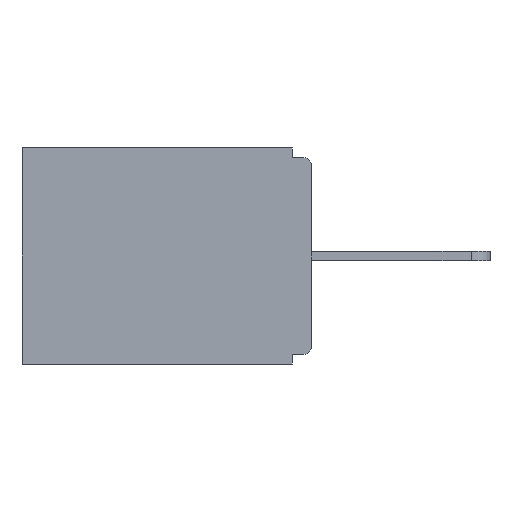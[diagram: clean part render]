
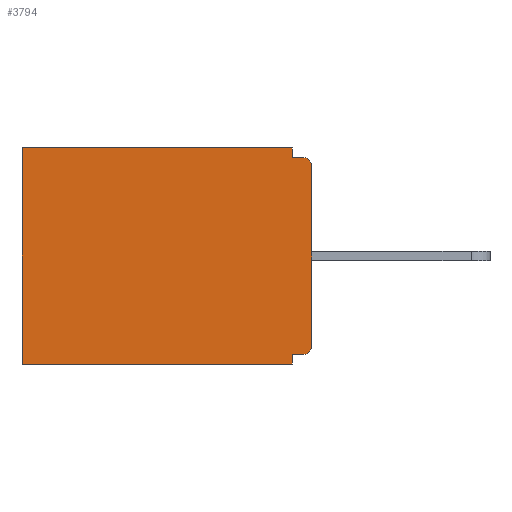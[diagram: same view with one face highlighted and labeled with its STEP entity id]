
A CAD part, left-side view. The second image highlights one B-rep face of the part: STEP entity #3794.
In plain terms, the highlighted planar face has unit normal (-1, 0, 0).
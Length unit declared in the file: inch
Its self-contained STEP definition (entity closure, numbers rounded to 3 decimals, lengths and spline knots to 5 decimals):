
#25 = EDGE_CURVE ( 'NONE', #3244, #3449, #8507, .T. ) ;
#71 = EDGE_CURVE ( 'NONE', #2868, #3944, #8250, .T. ) ;
#76 = EDGE_CURVE ( 'NONE', #2748, #3449, #305, .T. ) ;
#212 = VECTOR ( 'NONE', #11504, 39.37008 ) ;
#305 = CIRCLE ( 'NONE', #8914, 0.015 ) ;
#352 = EDGE_CURVE ( 'NONE', #10212, #10152, #7725, .T. ) ;
#494 = CARTESIAN_POINT ( 'NONE',  ( 0.298, 0., -0.03 ) ) ;
#547 = ORIENTED_EDGE ( 'NONE', *, *, #9572, .F. ) ;
#692 = EDGE_CURVE ( 'NONE', #7930, #3244, #10405, .T. ) ;
#705 = CARTESIAN_POINT ( 'NONE',  ( 0.298, 0.015, -0.015 ) ) ;
#718 = EDGE_CURVE ( 'NONE', #8031, #10212, #5612, .T. ) ;
#970 = AXIS2_PLACEMENT_3D ( 'NONE', #11041, #10339, #5010 ) ;
#1427 = EDGE_CURVE ( 'NONE', #2748, #3944, #3379, .T. ) ;
#1554 = ORIENTED_EDGE ( 'NONE', *, *, #352, .F. ) ;
#1727 = LINE ( 'NONE', #11512, #6712 ) ;
#1732 = ORIENTED_EDGE ( 'NONE', *, *, #71, .T. ) ;
#2217 = DIRECTION ( 'NONE',  ( 0., 0., -1. ) ) ;
#2494 = ORIENTED_EDGE ( 'NONE', *, *, #692, .F. ) ;
#2748 = VERTEX_POINT ( 'NONE', #494 ) ;
#2868 = VERTEX_POINT ( 'NONE', #10251 ) ;
#3238 = VECTOR ( 'NONE', #11605, 39.37008 ) ;
#3244 = VERTEX_POINT ( 'NONE', #5367 ) ;
#3320 = ORIENTED_EDGE ( 'NONE', *, *, #1427, .F. ) ;
#3379 = LINE ( 'NONE', #7099, #212 ) ;
#3441 = DIRECTION ( 'NONE',  ( 0., 0., -1. ) ) ;
#3449 = VERTEX_POINT ( 'NONE', #705 ) ;
#3635 = FACE_OUTER_BOUND ( 'NONE', #6264, .T. ) ;
#3721 = EDGE_CURVE ( 'NONE', #7930, #6276, #11549, .T. ) ;
#3794 = ADVANCED_FACE ( 'NONE', ( #3635 ), #8223, .F. ) ;
#3944 = VERTEX_POINT ( 'NONE', #6738 ) ;
#4465 = DIRECTION ( 'NONE',  ( 0., 1., 0. ) ) ;
#4669 = DIRECTION ( 'NONE',  ( -1., 0., 0. ) ) ;
#4845 = VECTOR ( 'NONE', #4465, 39.37008 ) ;
#5010 = DIRECTION ( 'NONE',  ( 0., 0., -1. ) ) ;
#5367 = CARTESIAN_POINT ( 'NONE',  ( 0.298, 0.031, -0.015 ) ) ;
#5612 = LINE ( 'NONE', #8700, #7573 ) ;
#5934 = CARTESIAN_POINT ( 'NONE',  ( 0.298, 0.031, -0.328 ) ) ;
#5972 = ORIENTED_EDGE ( 'NONE', *, *, #3721, .T. ) ;
#6064 = ORIENTED_EDGE ( 'NONE', *, *, #76, .T. ) ;
#6264 = EDGE_LOOP ( 'NONE', ( #6064, #11234, #2494, #5972, #8966, #1554, #6374, #547, #1732, #3320 ) ) ;
#6276 = VERTEX_POINT ( 'NONE', #7343 ) ;
#6374 = ORIENTED_EDGE ( 'NONE', *, *, #718, .F. ) ;
#6421 = CARTESIAN_POINT ( 'NONE',  ( 0.298, 0.031, -0.343 ) ) ;
#6712 = VECTOR ( 'NONE', #3441, 39.37008 ) ;
#6738 = CARTESIAN_POINT ( 'NONE',  ( 0.298, 0., -0.313 ) ) ;
#6954 = DIRECTION ( 'NONE',  ( 0., -1., 0. ) ) ;
#7099 = CARTESIAN_POINT ( 'NONE',  ( 0.298, 0., 0. ) ) ;
#7343 = CARTESIAN_POINT ( 'NONE',  ( 0.298, 0.46, 0. ) ) ;
#7573 = VECTOR ( 'NONE', #11010, 39.37008 ) ;
#7607 = CARTESIAN_POINT ( 'NONE',  ( 0.298, 0., 0. ) ) ;
#7619 = DIRECTION ( 'NONE',  ( 0., 0., -1. ) ) ;
#7674 = CARTESIAN_POINT ( 'NONE',  ( 0.298, 0.015, -0.313 ) ) ;
#7725 = LINE ( 'NONE', #11354, #7980 ) ;
#7837 = CARTESIAN_POINT ( 'NONE',  ( 0.298, 0.031, -0.343 ) ) ;
#7930 = VERTEX_POINT ( 'NONE', #10557 ) ;
#7980 = VECTOR ( 'NONE', #11092, 39.37008 ) ;
#8031 = VERTEX_POINT ( 'NONE', #5934 ) ;
#8187 = CARTESIAN_POINT ( 'NONE',  ( 0.298, 0.015, -0.03 ) ) ;
#8223 = PLANE ( 'NONE',  #970 ) ;
#8250 = CIRCLE ( 'NONE', #8423, 0.015 ) ;
#8378 = EDGE_CURVE ( 'NONE', #6276, #10152, #1727, .T. ) ;
#8423 = AXIS2_PLACEMENT_3D ( 'NONE', #7674, #9381, #7619 ) ;
#8507 = LINE ( 'NONE', #10325, #10756 ) ;
#8700 = CARTESIAN_POINT ( 'NONE',  ( 0.298, 0.031, -0.343 ) ) ;
#8782 = CARTESIAN_POINT ( 'NONE',  ( 0.298, 0., -0.328 ) ) ;
#8914 = AXIS2_PLACEMENT_3D ( 'NONE', #8187, #4669, #2217 ) ;
#8939 = DIRECTION ( 'NONE',  ( 0., 1., 0. ) ) ;
#8966 = ORIENTED_EDGE ( 'NONE', *, *, #8378, .T. ) ;
#9381 = DIRECTION ( 'NONE',  ( -1., 0., 0. ) ) ;
#9572 = EDGE_CURVE ( 'NONE', #2868, #8031, #11200, .T. ) ;
#9645 = CARTESIAN_POINT ( 'NONE',  ( 0.298, 0.46, -0.343 ) ) ;
#10152 = VERTEX_POINT ( 'NONE', #9645 ) ;
#10212 = VERTEX_POINT ( 'NONE', #6421 ) ;
#10251 = CARTESIAN_POINT ( 'NONE',  ( 0.298, 0.015, -0.328 ) ) ;
#10325 = CARTESIAN_POINT ( 'NONE',  ( 0.298, 0., -0.015 ) ) ;
#10339 = DIRECTION ( 'NONE',  ( 1., 0., 0. ) ) ;
#10405 = LINE ( 'NONE', #7837, #3238 ) ;
#10557 = CARTESIAN_POINT ( 'NONE',  ( 0.298, 0.031, 0. ) ) ;
#10752 = VECTOR ( 'NONE', #8939, 39.37008 ) ;
#10756 = VECTOR ( 'NONE', #6954, 39.37008 ) ;
#11010 = DIRECTION ( 'NONE',  ( 0., 0., -1. ) ) ;
#11041 = CARTESIAN_POINT ( 'NONE',  ( 0.298, 0., 0. ) ) ;
#11092 = DIRECTION ( 'NONE',  ( 0., 1., 0. ) ) ;
#11200 = LINE ( 'NONE', #8782, #10752 ) ;
#11234 = ORIENTED_EDGE ( 'NONE', *, *, #25, .F. ) ;
#11354 = CARTESIAN_POINT ( 'NONE',  ( 0.298, 0., -0.343 ) ) ;
#11504 = DIRECTION ( 'NONE',  ( 0., 0., -1. ) ) ;
#11512 = CARTESIAN_POINT ( 'NONE',  ( 0.298, 0.46, 0. ) ) ;
#11549 = LINE ( 'NONE', #7607, #4845 ) ;
#11605 = DIRECTION ( 'NONE',  ( 0., 0., -1. ) ) ;
